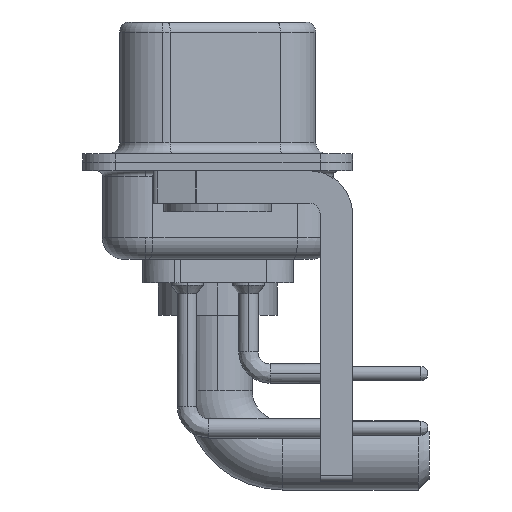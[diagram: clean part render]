
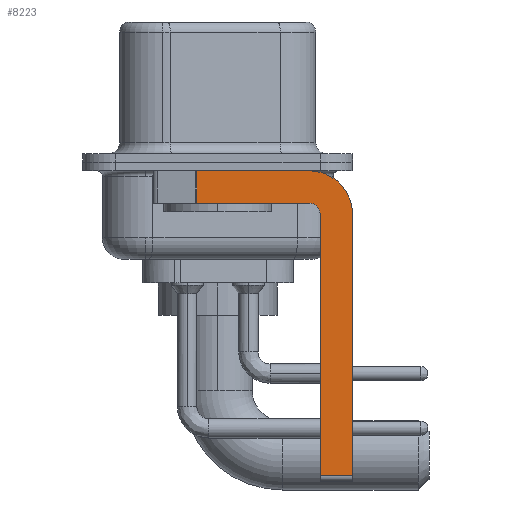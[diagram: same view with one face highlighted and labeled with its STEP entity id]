
A CAD part, left-side view. The second image highlights one B-rep face of the part: STEP entity #8223.
In plain terms, the highlighted planar face has unit normal (-1, 0, 0).
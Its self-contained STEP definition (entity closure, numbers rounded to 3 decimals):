
#1282 = DIRECTION ( 'NONE',  ( 0., 0., -1. ) ) ;
#2023 = ORIENTED_EDGE ( 'NONE', *, *, #15455, .F. ) ;
#2190 = DIRECTION ( 'NONE',  ( 0., 0., -1. ) ) ;
#2447 = CARTESIAN_POINT ( 'NONE',  ( -2.9, -4.25, -14.55 ) ) ;
#2465 = PLANE ( 'NONE',  #12200 ) ;
#2654 = DIRECTION ( 'NONE',  ( -1., 0., 0. ) ) ;
#2865 = VERTEX_POINT ( 'NONE', #17854 ) ;
#3076 = DIRECTION ( 'NONE',  ( 0., 0., -1. ) ) ;
#3173 = CARTESIAN_POINT ( 'NONE',  ( -2.9, -6.25, -2.4 ) ) ;
#3649 = VERTEX_POINT ( 'NONE', #5742 ) ;
#3825 = CARTESIAN_POINT ( 'NONE',  ( -2.9, -4.25, -1.9 ) ) ;
#4318 = LINE ( 'NONE', #10115, #19389 ) ;
#4552 = VECTOR ( 'NONE', #6432, 1000. ) ;
#4660 = EDGE_CURVE ( 'NONE', #10875, #5312, #4318, .T. ) ;
#4732 = LINE ( 'NONE', #2447, #9570 ) ;
#5312 = VERTEX_POINT ( 'NONE', #23038 ) ;
#5449 = ORIENTED_EDGE ( 'NONE', *, *, #13715, .T. ) ;
#5742 = CARTESIAN_POINT ( 'NONE',  ( -2.9, -6.25, -14.55 ) ) ;
#5889 = EDGE_CURVE ( 'NONE', #7076, #11148, #14664, .T. ) ;
#6419 = VECTOR ( 'NONE', #16143, 1000. ) ;
#6432 = DIRECTION ( 'NONE',  ( 0., -1., 0. ) ) ;
#6436 = CARTESIAN_POINT ( 'NONE',  ( -2.9, -4.25, -2.4 ) ) ;
#6541 = ORIENTED_EDGE ( 'NONE', *, *, #14439, .T. ) ;
#7076 = VERTEX_POINT ( 'NONE', #26394 ) ;
#7303 = EDGE_CURVE ( 'NONE', #24337, #10875, #11308, .T. ) ;
#7895 = LINE ( 'NONE', #16007, #6419 ) ;
#8223 = ADVANCED_FACE ( 'NONE', ( #22696 ), #2465, .F. ) ;
#8266 = ORIENTED_EDGE ( 'NONE', *, *, #7303, .F. ) ;
#8519 = DIRECTION ( 'NONE',  ( 1., 0., 0. ) ) ;
#9358 = VERTEX_POINT ( 'NONE', #3173 ) ;
#9570 = VECTOR ( 'NONE', #10925, 1000. ) ;
#10115 = CARTESIAN_POINT ( 'NONE',  ( -2.9, -4.25, -1.9 ) ) ;
#10456 = AXIS2_PLACEMENT_3D ( 'NONE', #11536, #19760, #1282 ) ;
#10875 = VERTEX_POINT ( 'NONE', #3825 ) ;
#10925 = DIRECTION ( 'NONE',  ( 0., -1., 0. ) ) ;
#11148 = VERTEX_POINT ( 'NONE', #13798 ) ;
#11308 = CIRCLE ( 'NONE', #24628, 0.5 ) ;
#11536 = CARTESIAN_POINT ( 'NONE',  ( -2.9, -4.25, -2.4 ) ) ;
#12200 = AXIS2_PLACEMENT_3D ( 'NONE', #16895, #8519, #2190 ) ;
#13715 = EDGE_CURVE ( 'NONE', #7076, #5312, #17506, .T. ) ;
#13798 = CARTESIAN_POINT ( 'NONE',  ( -2.9, -4.25, -0.4 ) ) ;
#14439 = EDGE_CURVE ( 'NONE', #2865, #3649, #4732, .T. ) ;
#14563 = CARTESIAN_POINT ( 'NONE',  ( -2.9, -4.75, -2.4 ) ) ;
#14664 = LINE ( 'NONE', #16693, #4552 ) ;
#14744 = LINE ( 'NONE', #14880, #24204 ) ;
#14880 = CARTESIAN_POINT ( 'NONE',  ( -2.9, -6.25, -2.4 ) ) ;
#14996 = ORIENTED_EDGE ( 'NONE', *, *, #25594, .F. ) ;
#15455 = EDGE_CURVE ( 'NONE', #11148, #9358, #22083, .T. ) ;
#16007 = CARTESIAN_POINT ( 'NONE',  ( -2.9, -4.75, -14.8 ) ) ;
#16143 = DIRECTION ( 'NONE',  ( 0., 0., 1. ) ) ;
#16165 = VECTOR ( 'NONE', #3076, 1000. ) ;
#16182 = ORIENTED_EDGE ( 'NONE', *, *, #18733, .F. ) ;
#16195 = DIRECTION ( 'NONE',  ( 0., 1., 0. ) ) ;
#16492 = DIRECTION ( 'NONE',  ( 0., 0., -1. ) ) ;
#16693 = CARTESIAN_POINT ( 'NONE',  ( -2.9, 3., -0.4 ) ) ;
#16895 = CARTESIAN_POINT ( 'NONE',  ( -2.9, -4.25, -2.4 ) ) ;
#17133 = ORIENTED_EDGE ( 'NONE', *, *, #4660, .F. ) ;
#17231 = CARTESIAN_POINT ( 'NONE',  ( -2.9, 0.978, -1.9 ) ) ;
#17506 = LINE ( 'NONE', #17231, #16165 ) ;
#17854 = CARTESIAN_POINT ( 'NONE',  ( -2.9, -4.75, -14.55 ) ) ;
#18733 = EDGE_CURVE ( 'NONE', #9358, #3649, #14744, .T. ) ;
#19389 = VECTOR ( 'NONE', #16195, 1000. ) ;
#19667 = EDGE_LOOP ( 'NONE', ( #21030, #5449, #17133, #8266, #14996, #6541, #16182, #2023 ) ) ;
#19760 = DIRECTION ( 'NONE',  ( 1., 0., 0. ) ) ;
#21002 = DIRECTION ( 'NONE',  ( 0., 0., 1. ) ) ;
#21030 = ORIENTED_EDGE ( 'NONE', *, *, #5889, .F. ) ;
#22083 = CIRCLE ( 'NONE', #10456, 2. ) ;
#22696 = FACE_OUTER_BOUND ( 'NONE', #19667, .T. ) ;
#23038 = CARTESIAN_POINT ( 'NONE',  ( -2.9, 0.978, -1.9 ) ) ;
#24204 = VECTOR ( 'NONE', #16492, 1000. ) ;
#24337 = VERTEX_POINT ( 'NONE', #14563 ) ;
#24628 = AXIS2_PLACEMENT_3D ( 'NONE', #6436, #2654, #21002 ) ;
#25594 = EDGE_CURVE ( 'NONE', #2865, #24337, #7895, .T. ) ;
#26394 = CARTESIAN_POINT ( 'NONE',  ( -2.9, 0.978, -0.4 ) ) ;
